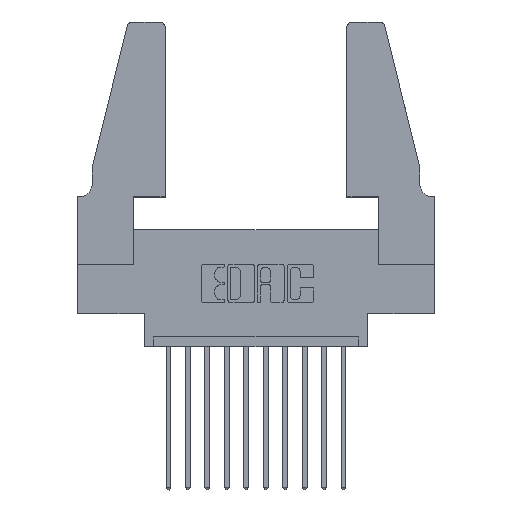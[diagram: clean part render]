
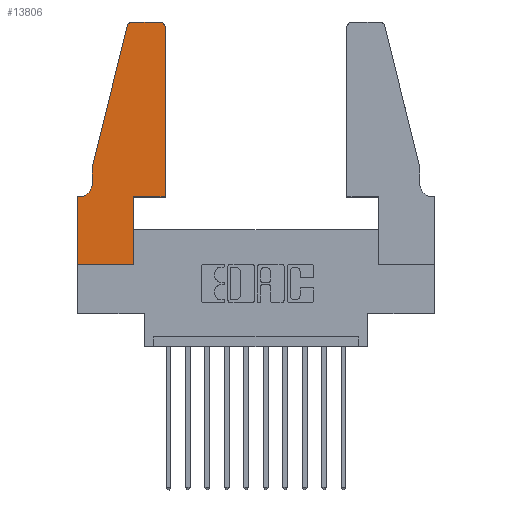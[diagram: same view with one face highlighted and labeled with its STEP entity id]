
A CAD part, top view. The second image highlights one B-rep face of the part: STEP entity #13806.
In plain terms, the highlighted planar face has unit normal (0, 0, 1).
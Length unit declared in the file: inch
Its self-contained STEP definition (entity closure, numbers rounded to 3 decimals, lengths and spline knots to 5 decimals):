
#156 = DIRECTION ( 'NONE',  ( 0., 0., 1. ) ) ;
#617 = LINE ( 'NONE', #12817, #8083 ) ;
#834 = CARTESIAN_POINT ( 'NONE',  ( 0., 0., 0.37 ) ) ;
#1120 = VERTEX_POINT ( 'NONE', #2043 ) ;
#1197 = DIRECTION ( 'NONE',  ( -0.239, -0.971, 0. ) ) ;
#1376 = VERTEX_POINT ( 'NONE', #10279 ) ;
#1383 = ORIENTED_EDGE ( 'NONE', *, *, #9450, .T. ) ;
#1558 = EDGE_CURVE ( 'NONE', #1120, #13569, #11638, .T. ) ;
#1644 = EDGE_CURVE ( 'NONE', #4093, #9399, #6490, .T. ) ;
#1646 = CARTESIAN_POINT ( 'NONE',  ( 0.0755, 0.5, 0.37 ) ) ;
#1944 = CARTESIAN_POINT ( 'NONE',  ( 0.284, 1.22, 0.37 ) ) ;
#2043 = CARTESIAN_POINT ( 'NONE',  ( 0.284, 1.25, 0.37 ) ) ;
#2168 = CARTESIAN_POINT ( 'NONE',  ( 0., 0.35, 0.37 ) ) ;
#2280 = CARTESIAN_POINT ( 'NONE',  ( 0.4505, 0.35, 0.37 ) ) ;
#2459 = CARTESIAN_POINT ( 'NONE',  ( 0.4205, 1.25, 0.37 ) ) ;
#2551 = LINE ( 'NONE', #11569, #10220 ) ;
#3197 = VECTOR ( 'NONE', #3975, 39.37008 ) ;
#3372 = EDGE_LOOP ( 'NONE', ( #13503, #4482, #13370, #6384, #8237, #1383, #10977, #4057, #6781, #5534, #10779, #8305 ) ) ;
#3855 = DIRECTION ( 'NONE',  ( 0., -1., 0. ) ) ;
#3975 = DIRECTION ( 'NONE',  ( -1., 0., 0. ) ) ;
#4057 = ORIENTED_EDGE ( 'NONE', *, *, #7978, .T. ) ;
#4093 = VERTEX_POINT ( 'NONE', #2280 ) ;
#4482 = ORIENTED_EDGE ( 'NONE', *, *, #1558, .T. ) ;
#4595 = EDGE_CURVE ( 'NONE', #6793, #4093, #13442, .T. ) ;
#4714 = LINE ( 'NONE', #9360, #5081 ) ;
#4726 = DIRECTION ( 'NONE',  ( 0., 0., -1. ) ) ;
#4740 = CARTESIAN_POINT ( 'NONE',  ( 0.4505, 1.22, 0.37 ) ) ;
#5081 = VECTOR ( 'NONE', #3855, 39.37008 ) ;
#5136 = VECTOR ( 'NONE', #9959, 39.37008 ) ;
#5147 = DIRECTION ( 'NONE',  ( 1., 0., 0. ) ) ;
#5216 = VECTOR ( 'NONE', #1197, 39.37008 ) ;
#5516 = CARTESIAN_POINT ( 'NONE',  ( 0.4505, 0.35, 0.37 ) ) ;
#5534 = ORIENTED_EDGE ( 'NONE', *, *, #4595, .T. ) ;
#5554 = EDGE_CURVE ( 'NONE', #1376, #6793, #617, .T. ) ;
#5589 = CARTESIAN_POINT ( 'NONE',  ( 0.0755, 0.5, 0.37 ) ) ;
#5646 = AXIS2_PLACEMENT_3D ( 'NONE', #10387, #4726, #7095 ) ;
#5704 = DIRECTION ( 'NONE',  ( 0., 0., 1. ) ) ;
#5797 = DIRECTION ( 'NONE',  ( 1., 0., 0. ) ) ;
#5863 = LINE ( 'NONE', #9392, #9439 ) ;
#6012 = CARTESIAN_POINT ( 'NONE',  ( 0.2865, 0.35, 0.37 ) ) ;
#6249 = VERTEX_POINT ( 'NONE', #2459 ) ;
#6342 = DIRECTION ( 'NONE',  ( 1., 0., 0. ) ) ;
#6384 = ORIENTED_EDGE ( 'NONE', *, *, #10102, .T. ) ;
#6490 = LINE ( 'NONE', #5516, #5136 ) ;
#6781 = ORIENTED_EDGE ( 'NONE', *, *, #5554, .T. ) ;
#6793 = VERTEX_POINT ( 'NONE', #6012 ) ;
#6982 = FACE_OUTER_BOUND ( 'NONE', #3372, .T. ) ;
#7095 = DIRECTION ( 'NONE',  ( -1., 0., 0. ) ) ;
#7110 = LINE ( 'NONE', #9390, #3197 ) ;
#7277 = VECTOR ( 'NONE', #7534, 39.37008 ) ;
#7352 = DIRECTION ( 'NONE',  ( 0., 0., 1. ) ) ;
#7534 = DIRECTION ( 'NONE',  ( 1., 0., 0. ) ) ;
#7739 = DIRECTION ( 'NONE',  ( 1., 0., 0. ) ) ;
#7859 = CARTESIAN_POINT ( 'NONE',  ( 0.4205, 1.22, 0.37 ) ) ;
#7978 = EDGE_CURVE ( 'NONE', #11544, #1376, #9584, .T. ) ;
#8083 = VECTOR ( 'NONE', #9925, 39.37008 ) ;
#8176 = DIRECTION ( 'NONE',  ( 0., -1., 0. ) ) ;
#8237 = ORIENTED_EDGE ( 'NONE', *, *, #10457, .T. ) ;
#8305 = ORIENTED_EDGE ( 'NONE', *, *, #13123, .T. ) ;
#8948 = CARTESIAN_POINT ( 'NONE',  ( 0., 0., 0.37 ) ) ;
#9360 = CARTESIAN_POINT ( 'NONE',  ( 0.0755, 0.5, 0.37 ) ) ;
#9390 = CARTESIAN_POINT ( 'NONE',  ( 0.0755, 0.35, 0.37 ) ) ;
#9392 = CARTESIAN_POINT ( 'NONE',  ( 0.2605, 1.25, 0.37 ) ) ;
#9399 = VERTEX_POINT ( 'NONE', #4740 ) ;
#9439 = VECTOR ( 'NONE', #11531, 39.37008 ) ;
#9441 = CARTESIAN_POINT ( 'NONE',  ( 0.25487, 1.22718, 0.37 ) ) ;
#9450 = EDGE_CURVE ( 'NONE', #11958, #11723, #7110, .T. ) ;
#9584 = LINE ( 'NONE', #8948, #11680 ) ;
#9925 = DIRECTION ( 'NONE',  ( 0., 1., 0. ) ) ;
#9959 = DIRECTION ( 'NONE',  ( 0., 1., 0. ) ) ;
#10102 = EDGE_CURVE ( 'NONE', #12973, #11792, #4714, .T. ) ;
#10220 = VECTOR ( 'NONE', #8176, 39.37008 ) ;
#10279 = CARTESIAN_POINT ( 'NONE',  ( 0.2865, 0., 0.37 ) ) ;
#10311 = AXIS2_PLACEMENT_3D ( 'NONE', #7859, #5704, #5797 ) ;
#10387 = CARTESIAN_POINT ( 'NONE',  ( 0.0055, 0.42, 0.37 ) ) ;
#10457 = EDGE_CURVE ( 'NONE', #11792, #11958, #11364, .T. ) ;
#10506 = AXIS2_PLACEMENT_3D ( 'NONE', #13216, #156, #7739 ) ;
#10739 = CARTESIAN_POINT ( 'NONE',  ( 0.0755, 0.42, 0.37 ) ) ;
#10779 = ORIENTED_EDGE ( 'NONE', *, *, #1644, .T. ) ;
#10841 = CARTESIAN_POINT ( 'NONE',  ( 0.4505, 0.35, 0.37 ) ) ;
#10977 = ORIENTED_EDGE ( 'NONE', *, *, #14055, .T. ) ;
#11103 = CIRCLE ( 'NONE', #10311, 0.03 ) ;
#11129 = EDGE_CURVE ( 'NONE', #13569, #12973, #14086, .T. ) ;
#11203 = CARTESIAN_POINT ( 'NONE',  ( 0.0055, 0.35, 0.37 ) ) ;
#11337 = AXIS2_PLACEMENT_3D ( 'NONE', #1944, #7352, #5147 ) ;
#11364 = CIRCLE ( 'NONE', #5646, 0.07 ) ;
#11531 = DIRECTION ( 'NONE',  ( -1., 0., 0. ) ) ;
#11544 = VERTEX_POINT ( 'NONE', #834 ) ;
#11569 = CARTESIAN_POINT ( 'NONE',  ( 0., 0., 0.37 ) ) ;
#11606 = EDGE_CURVE ( 'NONE', #6249, #1120, #5863, .T. ) ;
#11638 = CIRCLE ( 'NONE', #11337, 0.03 ) ;
#11680 = VECTOR ( 'NONE', #6342, 39.37008 ) ;
#11723 = VERTEX_POINT ( 'NONE', #2168 ) ;
#11792 = VERTEX_POINT ( 'NONE', #10739 ) ;
#11958 = VERTEX_POINT ( 'NONE', #11203 ) ;
#12144 = PLANE ( 'NONE',  #10506 ) ;
#12817 = CARTESIAN_POINT ( 'NONE',  ( 0.2865, 0.35, 0.37 ) ) ;
#12973 = VERTEX_POINT ( 'NONE', #1646 ) ;
#13123 = EDGE_CURVE ( 'NONE', #9399, #6249, #11103, .T. ) ;
#13216 = CARTESIAN_POINT ( 'NONE',  ( 0., 0.35, 0.37 ) ) ;
#13370 = ORIENTED_EDGE ( 'NONE', *, *, #11129, .T. ) ;
#13442 = LINE ( 'NONE', #10841, #7277 ) ;
#13503 = ORIENTED_EDGE ( 'NONE', *, *, #11606, .T. ) ;
#13569 = VERTEX_POINT ( 'NONE', #9441 ) ;
#13806 = ADVANCED_FACE ( 'NONE', ( #6982 ), #12144, .T. ) ;
#14055 = EDGE_CURVE ( 'NONE', #11723, #11544, #2551, .T. ) ;
#14086 = LINE ( 'NONE', #5589, #5216 ) ;
